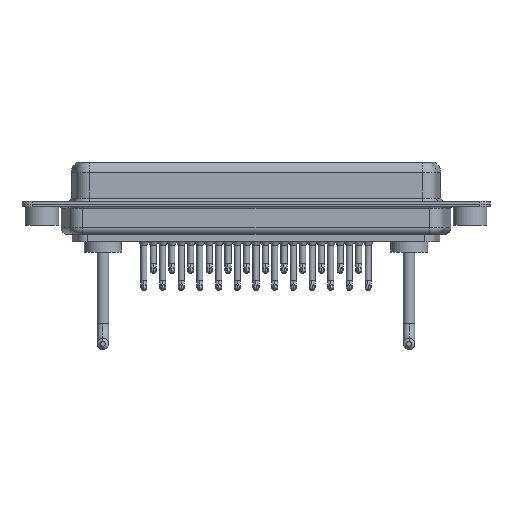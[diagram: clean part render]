
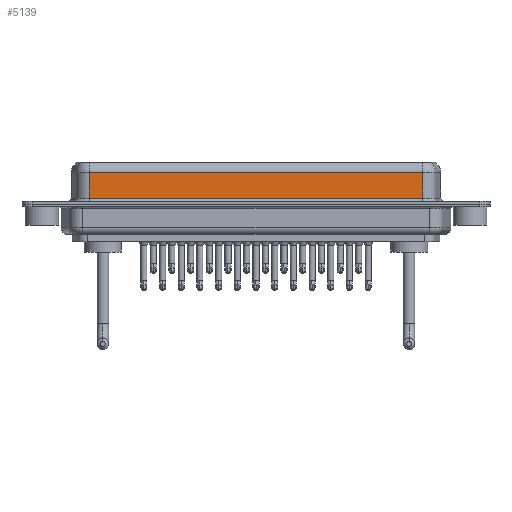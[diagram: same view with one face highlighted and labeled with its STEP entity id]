
A CAD part, front view. The second image highlights one B-rep face of the part: STEP entity #5139.
In plain terms, the highlighted planar face has unit normal (0, -1, 0).
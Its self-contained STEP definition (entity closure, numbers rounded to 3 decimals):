
#397 = CARTESIAN_POINT ( 'NONE',  ( 7.038, -3.95, 4.65 ) ) ;
#417 = EDGE_LOOP ( 'NONE', ( #5110, #16227, #4857, #19786 ) ) ;
#512 = LINE ( 'NONE', #7913, #3051 ) ;
#2624 = CARTESIAN_POINT ( 'NONE',  ( 56.462, -3.95, 4.65 ) ) ;
#3051 = VECTOR ( 'NONE', #5900, 1000. ) ;
#3314 = DIRECTION ( 'NONE',  ( 1., 0., 0. ) ) ;
#3412 = VERTEX_POINT ( 'NONE', #397 ) ;
#4430 = EDGE_CURVE ( 'NONE', #24151, #7895, #14665, .T. ) ;
#4857 = ORIENTED_EDGE ( 'NONE', *, *, #10073, .T. ) ;
#4930 = VERTEX_POINT ( 'NONE', #24287 ) ;
#5110 = ORIENTED_EDGE ( 'NONE', *, *, #4430, .F. ) ;
#5139 = ADVANCED_FACE ( 'NONE', ( #16983 ), #24643, .F. ) ;
#5847 = CARTESIAN_POINT ( 'NONE',  ( 56.462, -3.95, 0.9 ) ) ;
#5900 = DIRECTION ( 'NONE',  ( -1., 0., 0. ) ) ;
#6122 = LINE ( 'NONE', #17517, #23690 ) ;
#6962 = CARTESIAN_POINT ( 'NONE',  ( 56.462, -3.95, 0.9 ) ) ;
#7146 = DIRECTION ( 'NONE',  ( 0., 0., -1. ) ) ;
#7895 = VERTEX_POINT ( 'NONE', #5847 ) ;
#7913 = CARTESIAN_POINT ( 'NONE',  ( 56.462, -3.95, 4.65 ) ) ;
#7959 = DIRECTION ( 'NONE',  ( 0., 0., 1. ) ) ;
#9778 = DIRECTION ( 'NONE',  ( 0., 0., -1. ) ) ;
#10073 = EDGE_CURVE ( 'NONE', #3412, #4930, #6122, .T. ) ;
#13025 = CARTESIAN_POINT ( 'NONE',  ( 56.462, -3.95, 6.4 ) ) ;
#14665 = LINE ( 'NONE', #13025, #16837 ) ;
#16227 = ORIENTED_EDGE ( 'NONE', *, *, #18874, .T. ) ;
#16837 = VECTOR ( 'NONE', #7146, 1000. ) ;
#16983 = FACE_OUTER_BOUND ( 'NONE', #417, .T. ) ;
#17104 = CARTESIAN_POINT ( 'NONE',  ( 56.462, -3.95, 6.4 ) ) ;
#17517 = CARTESIAN_POINT ( 'NONE',  ( 7.038, -3.95, 6.4 ) ) ;
#17697 = EDGE_CURVE ( 'NONE', #4930, #7895, #20495, .T. ) ;
#18874 = EDGE_CURVE ( 'NONE', #24151, #3412, #512, .T. ) ;
#19786 = ORIENTED_EDGE ( 'NONE', *, *, #17697, .T. ) ;
#20495 = LINE ( 'NONE', #6962, #20814 ) ;
#20814 = VECTOR ( 'NONE', #3314, 1000. ) ;
#20891 = DIRECTION ( 'NONE',  ( 0., 1., 0. ) ) ;
#23690 = VECTOR ( 'NONE', #9778, 1000. ) ;
#24077 = AXIS2_PLACEMENT_3D ( 'NONE', #17104, #20891, #7959 ) ;
#24151 = VERTEX_POINT ( 'NONE', #2624 ) ;
#24287 = CARTESIAN_POINT ( 'NONE',  ( 7.038, -3.95, 0.9 ) ) ;
#24643 = PLANE ( 'NONE',  #24077 ) ;
